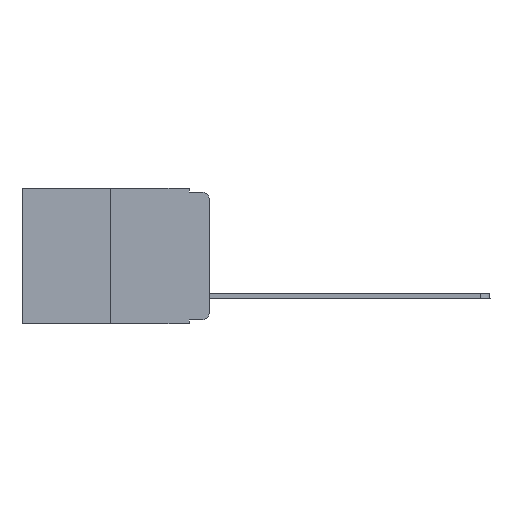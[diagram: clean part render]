
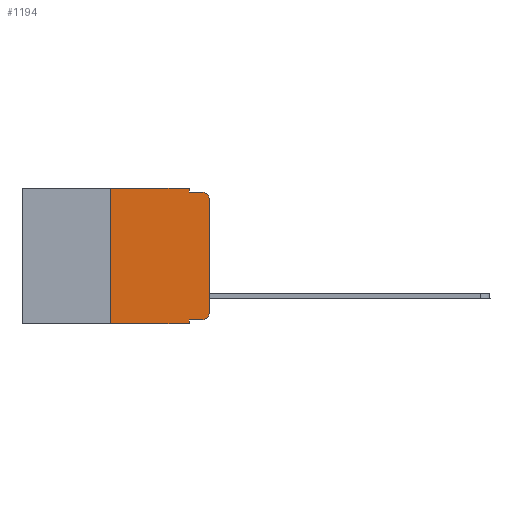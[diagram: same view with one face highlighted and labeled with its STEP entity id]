
A CAD part, left-side view. The second image highlights one B-rep face of the part: STEP entity #1194.
In plain terms, the highlighted planar face has unit normal (-1, 0, 0).
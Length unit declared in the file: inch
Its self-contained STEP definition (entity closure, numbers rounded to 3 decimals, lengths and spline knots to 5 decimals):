
#275 = ORIENTED_EDGE ( 'NONE', *, *, #7265, .F. ) ;
#317 = VECTOR ( 'NONE', #3970, 39.37008 ) ;
#740 = ORIENTED_EDGE ( 'NONE', *, *, #2633, .F. ) ;
#768 = CARTESIAN_POINT ( 'NONE',  ( 0., 0.051, 0. ) ) ;
#879 = VECTOR ( 'NONE', #13501, 39.37008 ) ;
#884 = EDGE_CURVE ( 'NONE', #5807, #15221, #17685, .T. ) ;
#931 = LINE ( 'NONE', #11017, #12077 ) ;
#955 = DIRECTION ( 'NONE',  ( 0., -1., 0. ) ) ;
#1104 = CARTESIAN_POINT ( 'NONE',  ( 0., 0.02, -0.01 ) ) ;
#1194 = ADVANCED_FACE ( 'NONE', ( #7856 ), #1608, .F. ) ;
#1245 = CARTESIAN_POINT ( 'NONE',  ( 0., 0., 0. ) ) ;
#1251 = EDGE_CURVE ( 'NONE', #4587, #2306, #8721, .T. ) ;
#1608 = PLANE ( 'NONE',  #9213 ) ;
#1623 = AXIS2_PLACEMENT_3D ( 'NONE', #8259, #13990, #5579 ) ;
#1871 = DIRECTION ( 'NONE',  ( 0., 0., -1. ) ) ;
#2306 = VERTEX_POINT ( 'NONE', #3871 ) ;
#2432 = VECTOR ( 'NONE', #955, 39.37008 ) ;
#2633 = EDGE_CURVE ( 'NONE', #7985, #13417, #931, .T. ) ;
#2811 = ORIENTED_EDGE ( 'NONE', *, *, #5841, .T. ) ;
#2846 = LINE ( 'NONE', #7945, #2432 ) ;
#3852 = CARTESIAN_POINT ( 'NONE',  ( 0., 0., -0.313 ) ) ;
#3871 = CARTESIAN_POINT ( 'NONE',  ( 0., 0.051, -0.01 ) ) ;
#3970 = DIRECTION ( 'NONE',  ( 0., 0., -1. ) ) ;
#4047 = LINE ( 'NONE', #6674, #317 ) ;
#4067 = EDGE_CURVE ( 'NONE', #11073, #16566, #5002, .T. ) ;
#4166 = AXIS2_PLACEMENT_3D ( 'NONE', #15815, #7370, #1871 ) ;
#4489 = EDGE_CURVE ( 'NONE', #13417, #4587, #7177, .T. ) ;
#4587 = VERTEX_POINT ( 'NONE', #768 ) ;
#4596 = EDGE_CURVE ( 'NONE', #7985, #13214, #2846, .T. ) ;
#5002 = LINE ( 'NONE', #10561, #11149 ) ;
#5235 = VECTOR ( 'NONE', #15830, 39.37008 ) ;
#5579 = DIRECTION ( 'NONE',  ( 0., 0., -1. ) ) ;
#5594 = DIRECTION ( 'NONE',  ( 0., 0., 1. ) ) ;
#5807 = VERTEX_POINT ( 'NONE', #15274 ) ;
#5841 = EDGE_CURVE ( 'NONE', #12834, #5807, #12202, .T. ) ;
#6029 = CARTESIAN_POINT ( 'NONE',  ( 0., 0.051, -0.333 ) ) ;
#6607 = CARTESIAN_POINT ( 'NONE',  ( 0., 0.051, -0.01 ) ) ;
#6674 = CARTESIAN_POINT ( 'NONE',  ( 0., 0.051, 0. ) ) ;
#7142 = EDGE_LOOP ( 'NONE', ( #2811, #15233, #15321, #9388, #14551, #740, #10897, #275, #12990, #16124 ) ) ;
#7177 = LINE ( 'NONE', #13312, #5235 ) ;
#7179 = LINE ( 'NONE', #6607, #879 ) ;
#7191 = VECTOR ( 'NONE', #10021, 39.37008 ) ;
#7244 = DIRECTION ( 'NONE',  ( 1., 0., 0. ) ) ;
#7265 = EDGE_CURVE ( 'NONE', #11073, #13214, #4047, .T. ) ;
#7370 = DIRECTION ( 'NONE',  ( -1., 0., 0. ) ) ;
#7632 = EDGE_CURVE ( 'NONE', #16566, #12834, #13232, .T. ) ;
#7656 = DIRECTION ( 'NONE',  ( 0., -1., 0. ) ) ;
#7856 = FACE_OUTER_BOUND ( 'NONE', #7142, .T. ) ;
#7945 = CARTESIAN_POINT ( 'NONE',  ( 0., 0.473, -0.343 ) ) ;
#7985 = VERTEX_POINT ( 'NONE', #13950 ) ;
#8259 = CARTESIAN_POINT ( 'NONE',  ( 0., 0.02, -0.03 ) ) ;
#8721 = LINE ( 'NONE', #11507, #7191 ) ;
#8876 = VECTOR ( 'NONE', #16682, 39.37008 ) ;
#9213 = AXIS2_PLACEMENT_3D ( 'NONE', #12911, #7244, #16861 ) ;
#9388 = ORIENTED_EDGE ( 'NONE', *, *, #1251, .F. ) ;
#10021 = DIRECTION ( 'NONE',  ( 0., 0., -1. ) ) ;
#10451 = CARTESIAN_POINT ( 'NONE',  ( 0., 0.25, 0. ) ) ;
#10561 = CARTESIAN_POINT ( 'NONE',  ( 0., 0.051, -0.333 ) ) ;
#10897 = ORIENTED_EDGE ( 'NONE', *, *, #4596, .T. ) ;
#11017 = CARTESIAN_POINT ( 'NONE',  ( 0., 0.25, 0. ) ) ;
#11073 = VERTEX_POINT ( 'NONE', #6029 ) ;
#11143 = CARTESIAN_POINT ( 'NONE',  ( 0., 0.02, -0.333 ) ) ;
#11149 = VECTOR ( 'NONE', #7656, 39.37008 ) ;
#11507 = CARTESIAN_POINT ( 'NONE',  ( 0., 0.051, 0. ) ) ;
#12077 = VECTOR ( 'NONE', #5594, 39.37008 ) ;
#12202 = LINE ( 'NONE', #1245, #8876 ) ;
#12834 = VERTEX_POINT ( 'NONE', #3852 ) ;
#12867 = CARTESIAN_POINT ( 'NONE',  ( 0., 0.051, -0.343 ) ) ;
#12911 = CARTESIAN_POINT ( 'NONE',  ( 0., 0.473, 0. ) ) ;
#12990 = ORIENTED_EDGE ( 'NONE', *, *, #4067, .T. ) ;
#13214 = VERTEX_POINT ( 'NONE', #12867 ) ;
#13232 = CIRCLE ( 'NONE', #4166, 0.02 ) ;
#13312 = CARTESIAN_POINT ( 'NONE',  ( 0., 0.473, 0. ) ) ;
#13417 = VERTEX_POINT ( 'NONE', #10451 ) ;
#13501 = DIRECTION ( 'NONE',  ( 0., -1., 0. ) ) ;
#13568 = EDGE_CURVE ( 'NONE', #2306, #15221, #7179, .T. ) ;
#13950 = CARTESIAN_POINT ( 'NONE',  ( 0., 0.25, -0.343 ) ) ;
#13990 = DIRECTION ( 'NONE',  ( -1., 0., 0. ) ) ;
#14551 = ORIENTED_EDGE ( 'NONE', *, *, #4489, .F. ) ;
#15221 = VERTEX_POINT ( 'NONE', #1104 ) ;
#15233 = ORIENTED_EDGE ( 'NONE', *, *, #884, .T. ) ;
#15274 = CARTESIAN_POINT ( 'NONE',  ( 0., 0., -0.03 ) ) ;
#15321 = ORIENTED_EDGE ( 'NONE', *, *, #13568, .F. ) ;
#15815 = CARTESIAN_POINT ( 'NONE',  ( 0., 0.02, -0.313 ) ) ;
#15830 = DIRECTION ( 'NONE',  ( 0., -1., 0. ) ) ;
#16124 = ORIENTED_EDGE ( 'NONE', *, *, #7632, .T. ) ;
#16566 = VERTEX_POINT ( 'NONE', #11143 ) ;
#16682 = DIRECTION ( 'NONE',  ( 0., 0., 1. ) ) ;
#16861 = DIRECTION ( 'NONE',  ( 0., 0., -1. ) ) ;
#17685 = CIRCLE ( 'NONE', #1623, 0.02 ) ;
